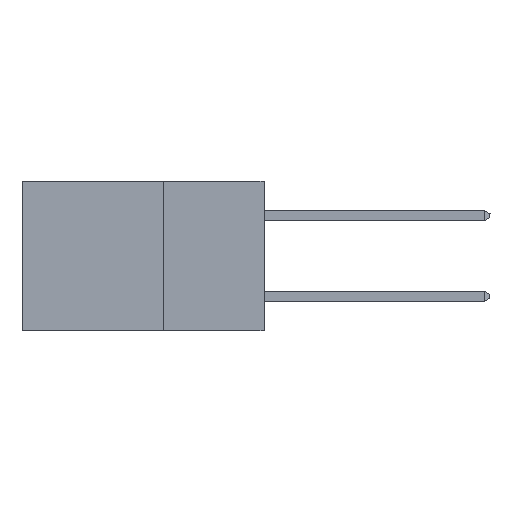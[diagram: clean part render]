
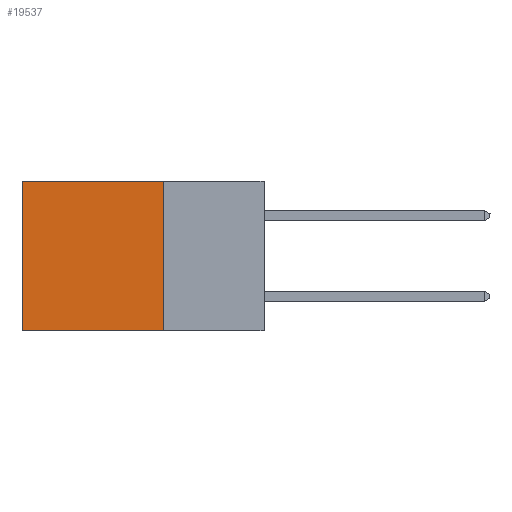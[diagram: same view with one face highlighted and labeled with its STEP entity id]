
A CAD part, left-side view. The second image highlights one B-rep face of the part: STEP entity #19537.
In plain terms, the highlighted planar face has unit normal (-1, 0, 0).
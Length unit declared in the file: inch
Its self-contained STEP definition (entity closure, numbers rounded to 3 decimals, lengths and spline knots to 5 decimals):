
#2504 = DIRECTION ( 'NONE',  ( 0., 0., -1. ) ) ;
#2857 = ORIENTED_EDGE ( 'NONE', *, *, #15991, .T. ) ;
#3109 = DIRECTION ( 'NONE',  ( 0., 0., -1. ) ) ;
#5936 = VERTEX_POINT ( 'NONE', #10306 ) ;
#8688 = LINE ( 'NONE', #18399, #18862 ) ;
#8873 = CARTESIAN_POINT ( 'NONE',  ( 0.298, 0.6, 0. ) ) ;
#9743 = ORIENTED_EDGE ( 'NONE', *, *, #25498, .F. ) ;
#9945 = CARTESIAN_POINT ( 'NONE',  ( 0.298, 0.25, 0. ) ) ;
#9998 = ORIENTED_EDGE ( 'NONE', *, *, #13330, .F. ) ;
#10306 = CARTESIAN_POINT ( 'NONE',  ( 0.298, 0.6, -0.37 ) ) ;
#10988 = VERTEX_POINT ( 'NONE', #8873 ) ;
#11796 = EDGE_CURVE ( 'NONE', #31338, #10988, #31849, .T. ) ;
#12635 = VECTOR ( 'NONE', #3109, 39.37008 ) ;
#13330 = EDGE_CURVE ( 'NONE', #31338, #19788, #24982, .T. ) ;
#14583 = DIRECTION ( 'NONE',  ( 0., 0., -1. ) ) ;
#15687 = DIRECTION ( 'NONE',  ( 0., 1., 0. ) ) ;
#15940 = AXIS2_PLACEMENT_3D ( 'NONE', #32345, #19361, #14583 ) ;
#15991 = EDGE_CURVE ( 'NONE', #10988, #5936, #30604, .T. ) ;
#18399 = CARTESIAN_POINT ( 'NONE',  ( 0.298, 0.25, -0.37 ) ) ;
#18430 = VECTOR ( 'NONE', #32116, 39.37008 ) ;
#18862 = VECTOR ( 'NONE', #15687, 39.37008 ) ;
#19125 = PLANE ( 'NONE',  #15940 ) ;
#19361 = DIRECTION ( 'NONE',  ( 1., 0., 0. ) ) ;
#19537 = ADVANCED_FACE ( 'NONE', ( #32780 ), #19125, .F. ) ;
#19788 = VERTEX_POINT ( 'NONE', #27859 ) ;
#19992 = ORIENTED_EDGE ( 'NONE', *, *, #11796, .T. ) ;
#23373 = EDGE_LOOP ( 'NONE', ( #2857, #9743, #9998, #19992 ) ) ;
#23460 = CARTESIAN_POINT ( 'NONE',  ( 0.298, 0.6, 0. ) ) ;
#24982 = LINE ( 'NONE', #28845, #12635 ) ;
#25288 = VECTOR ( 'NONE', #2504, 39.37008 ) ;
#25498 = EDGE_CURVE ( 'NONE', #19788, #5936, #8688, .T. ) ;
#27859 = CARTESIAN_POINT ( 'NONE',  ( 0.298, 0.25, -0.37 ) ) ;
#28800 = CARTESIAN_POINT ( 'NONE',  ( 0.298, 0.25, 0. ) ) ;
#28845 = CARTESIAN_POINT ( 'NONE',  ( 0.298, 0.25, 0. ) ) ;
#30604 = LINE ( 'NONE', #23460, #25288 ) ;
#31338 = VERTEX_POINT ( 'NONE', #9945 ) ;
#31849 = LINE ( 'NONE', #28800, #18430 ) ;
#32116 = DIRECTION ( 'NONE',  ( 0., 1., 0. ) ) ;
#32345 = CARTESIAN_POINT ( 'NONE',  ( 0.298, 0.25, 0. ) ) ;
#32780 = FACE_OUTER_BOUND ( 'NONE', #23373, .T. ) ;
